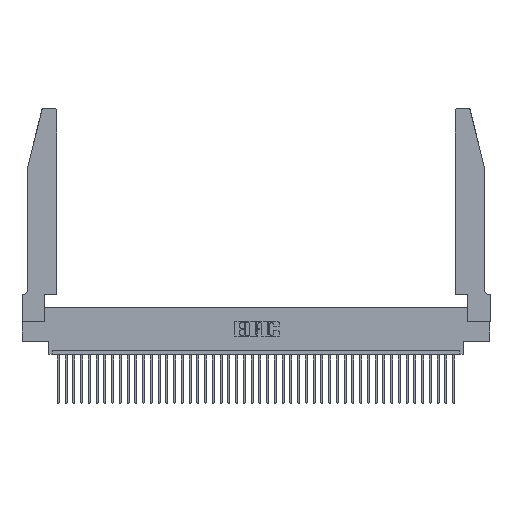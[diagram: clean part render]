
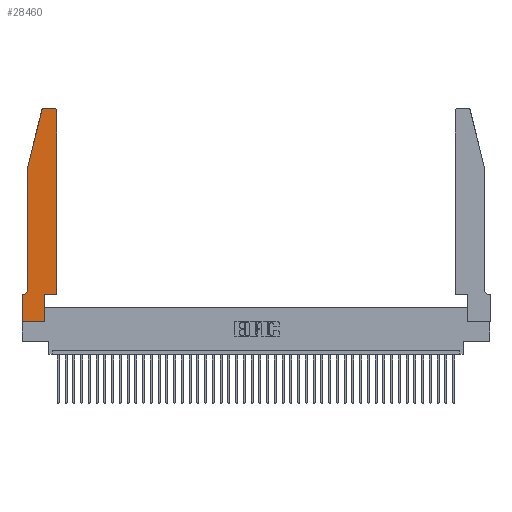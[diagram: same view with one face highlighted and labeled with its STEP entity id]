
A CAD part, top view. The second image highlights one B-rep face of the part: STEP entity #28460.
In plain terms, the highlighted planar face has unit normal (0, 0, 1).
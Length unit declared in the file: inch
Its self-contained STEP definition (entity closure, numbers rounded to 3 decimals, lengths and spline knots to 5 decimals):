
#626 = VECTOR ( 'NONE', #2468, 39.37008 ) ;
#741 = CARTESIAN_POINT ( 'NONE',  ( 0.2865, 0.35, 0.37 ) ) ;
#1520 = CARTESIAN_POINT ( 'NONE',  ( 0.25487, 2.72718, 0.37 ) ) ;
#1581 = VERTEX_POINT ( 'NONE', #6895 ) ;
#1720 = EDGE_CURVE ( 'NONE', #35896, #16081, #9621, .T. ) ;
#2281 = ORIENTED_EDGE ( 'NONE', *, *, #20594, .T. ) ;
#2468 = DIRECTION ( 'NONE',  ( -1., 0., 0. ) ) ;
#2874 = CARTESIAN_POINT ( 'NONE',  ( 0.4205, 2.72, 0.37 ) ) ;
#3200 = VERTEX_POINT ( 'NONE', #28444 ) ;
#3681 = DIRECTION ( 'NONE',  ( 1., 0., 0. ) ) ;
#4075 = DIRECTION ( 'NONE',  ( 0., 1., 0. ) ) ;
#5694 = EDGE_CURVE ( 'NONE', #16081, #37127, #31649, .T. ) ;
#6895 = CARTESIAN_POINT ( 'NONE',  ( 0.4205, 2.75, 0.37 ) ) ;
#7000 = EDGE_CURVE ( 'NONE', #3200, #22905, #19722, .T. ) ;
#7126 = ORIENTED_EDGE ( 'NONE', *, *, #42721, .T. ) ;
#7442 = LINE ( 'NONE', #34345, #40455 ) ;
#7716 = ORIENTED_EDGE ( 'NONE', *, *, #1720, .T. ) ;
#9230 = ORIENTED_EDGE ( 'NONE', *, *, #9305, .T. ) ;
#9277 = DIRECTION ( 'NONE',  ( 0., 0., 1. ) ) ;
#9305 = EDGE_CURVE ( 'NONE', #34108, #1581, #40645, .T. ) ;
#9547 = VECTOR ( 'NONE', #22609, 39.37008 ) ;
#9562 = ORIENTED_EDGE ( 'NONE', *, *, #41179, .T. ) ;
#9621 = CIRCLE ( 'NONE', #11774, 0.03 ) ;
#9993 = ORIENTED_EDGE ( 'NONE', *, *, #23415, .T. ) ;
#10461 = ORIENTED_EDGE ( 'NONE', *, *, #7000, .T. ) ;
#10945 = VECTOR ( 'NONE', #22620, 39.37008 ) ;
#11774 = AXIS2_PLACEMENT_3D ( 'NONE', #25150, #31698, #35037 ) ;
#12694 = DIRECTION ( 'NONE',  ( 1., 0., 0. ) ) ;
#13200 = CARTESIAN_POINT ( 'NONE',  ( 0.0755, 2., 0.37 ) ) ;
#13743 = CARTESIAN_POINT ( 'NONE',  ( 0.4505, 0.35, 0.37 ) ) ;
#14235 = EDGE_CURVE ( 'NONE', #22905, #27345, #7442, .T. ) ;
#15074 = DIRECTION ( 'NONE',  ( 0., 1., 0. ) ) ;
#15941 = AXIS2_PLACEMENT_3D ( 'NONE', #42116, #9277, #12694 ) ;
#16081 = VERTEX_POINT ( 'NONE', #1520 ) ;
#17200 = VERTEX_POINT ( 'NONE', #24335 ) ;
#17530 = DIRECTION ( 'NONE',  ( 1., 0., 0. ) ) ;
#17634 = CARTESIAN_POINT ( 'NONE',  ( 0.4505, 2.72, 0.37 ) ) ;
#18285 = ORIENTED_EDGE ( 'NONE', *, *, #40751, .T. ) ;
#18930 = DIRECTION ( 'NONE',  ( 0., -1., 0. ) ) ;
#19118 = VERTEX_POINT ( 'NONE', #41917 ) ;
#19319 = ORIENTED_EDGE ( 'NONE', *, *, #5694, .T. ) ;
#19722 = LINE ( 'NONE', #22336, #10945 ) ;
#20594 = EDGE_CURVE ( 'NONE', #27345, #17200, #39028, .T. ) ;
#21524 = VECTOR ( 'NONE', #4075, 39.37008 ) ;
#22269 = CARTESIAN_POINT ( 'NONE',  ( 0.0755, 0.35, 0.37 ) ) ;
#22322 = CARTESIAN_POINT ( 'NONE',  ( 0.2605, 2.75, 0.37 ) ) ;
#22336 = CARTESIAN_POINT ( 'NONE',  ( 0., 0., 0.37 ) ) ;
#22609 = DIRECTION ( 'NONE',  ( -0.239, -0.971, 0. ) ) ;
#22620 = DIRECTION ( 'NONE',  ( 0., -1., 0. ) ) ;
#22769 = VERTEX_POINT ( 'NONE', #30684 ) ;
#22838 = LINE ( 'NONE', #22269, #626 ) ;
#22905 = VERTEX_POINT ( 'NONE', #31697 ) ;
#22962 = FACE_OUTER_BOUND ( 'NONE', #33321, .T. ) ;
#23415 = EDGE_CURVE ( 'NONE', #19118, #22769, #41420, .T. ) ;
#23551 = LINE ( 'NONE', #27916, #36399 ) ;
#24010 = DIRECTION ( 'NONE',  ( 0., 0., -1. ) ) ;
#24152 = EDGE_CURVE ( 'NONE', #1581, #35896, #26456, .T. ) ;
#24335 = CARTESIAN_POINT ( 'NONE',  ( 0.2865, 0.35, 0.37 ) ) ;
#25150 = CARTESIAN_POINT ( 'NONE',  ( 0.284, 2.72, 0.37 ) ) ;
#25436 = VECTOR ( 'NONE', #42581, 39.37008 ) ;
#25456 = VECTOR ( 'NONE', #18930, 39.37008 ) ;
#26456 = LINE ( 'NONE', #22322, #25436 ) ;
#27345 = VERTEX_POINT ( 'NONE', #30808 ) ;
#27382 = ORIENTED_EDGE ( 'NONE', *, *, #14235, .T. ) ;
#27916 = CARTESIAN_POINT ( 'NONE',  ( 0.4505, 0.35, 0.37 ) ) ;
#28444 = CARTESIAN_POINT ( 'NONE',  ( 0., 0.35, 0.37 ) ) ;
#28460 = ADVANCED_FACE ( 'NONE', ( #22962 ), #28831, .T. ) ;
#28831 = PLANE ( 'NONE',  #15941 ) ;
#29413 = VECTOR ( 'NONE', #3681, 39.37008 ) ;
#30684 = CARTESIAN_POINT ( 'NONE',  ( 0.0055, 0.35, 0.37 ) ) ;
#30808 = CARTESIAN_POINT ( 'NONE',  ( 0.2865, 0., 0.37 ) ) ;
#31301 = ORIENTED_EDGE ( 'NONE', *, *, #24152, .T. ) ;
#31649 = LINE ( 'NONE', #38709, #9547 ) ;
#31697 = CARTESIAN_POINT ( 'NONE',  ( 0., 0., 0.37 ) ) ;
#31698 = DIRECTION ( 'NONE',  ( 0., 0., 1. ) ) ;
#31896 = EDGE_CURVE ( 'NONE', #37127, #19118, #34132, .T. ) ;
#33321 = EDGE_LOOP ( 'NONE', ( #31301, #7716, #19319, #39838, #9993, #7126, #10461, #27382, #2281, #9562, #18285, #9230 ) ) ;
#33730 = CARTESIAN_POINT ( 'NONE',  ( 0.0055, 0.42, 0.37 ) ) ;
#33878 = DIRECTION ( 'NONE',  ( -1., 0., 0. ) ) ;
#34108 = VERTEX_POINT ( 'NONE', #17634 ) ;
#34132 = LINE ( 'NONE', #36049, #25456 ) ;
#34204 = CARTESIAN_POINT ( 'NONE',  ( 0.284, 2.75, 0.37 ) ) ;
#34345 = CARTESIAN_POINT ( 'NONE',  ( 0., 0., 0.37 ) ) ;
#34549 = VERTEX_POINT ( 'NONE', #41133 ) ;
#35037 = DIRECTION ( 'NONE',  ( 1., 0., 0. ) ) ;
#35835 = DIRECTION ( 'NONE',  ( 0., 0., 1. ) ) ;
#35896 = VERTEX_POINT ( 'NONE', #34204 ) ;
#36049 = CARTESIAN_POINT ( 'NONE',  ( 0.0755, 2., 0.37 ) ) ;
#36399 = VECTOR ( 'NONE', #15074, 39.37008 ) ;
#37127 = VERTEX_POINT ( 'NONE', #13200 ) ;
#38709 = CARTESIAN_POINT ( 'NONE',  ( 0.0755, 2., 0.37 ) ) ;
#39028 = LINE ( 'NONE', #741, #21524 ) ;
#39583 = DIRECTION ( 'NONE',  ( 1., 0., 0. ) ) ;
#39838 = ORIENTED_EDGE ( 'NONE', *, *, #31896, .T. ) ;
#40341 = AXIS2_PLACEMENT_3D ( 'NONE', #33730, #24010, #33878 ) ;
#40455 = VECTOR ( 'NONE', #17530, 39.37008 ) ;
#40602 = AXIS2_PLACEMENT_3D ( 'NONE', #2874, #35835, #39583 ) ;
#40645 = CIRCLE ( 'NONE', #40602, 0.03 ) ;
#40751 = EDGE_CURVE ( 'NONE', #34549, #34108, #23551, .T. ) ;
#41133 = CARTESIAN_POINT ( 'NONE',  ( 0.4505, 0.35, 0.37 ) ) ;
#41179 = EDGE_CURVE ( 'NONE', #17200, #34549, #41326, .T. ) ;
#41326 = LINE ( 'NONE', #13743, #29413 ) ;
#41420 = CIRCLE ( 'NONE', #40341, 0.07 ) ;
#41917 = CARTESIAN_POINT ( 'NONE',  ( 0.0755, 0.42, 0.37 ) ) ;
#42116 = CARTESIAN_POINT ( 'NONE',  ( 0., 0.35, 0.37 ) ) ;
#42581 = DIRECTION ( 'NONE',  ( -1., 0., 0. ) ) ;
#42721 = EDGE_CURVE ( 'NONE', #22769, #3200, #22838, .T. ) ;
